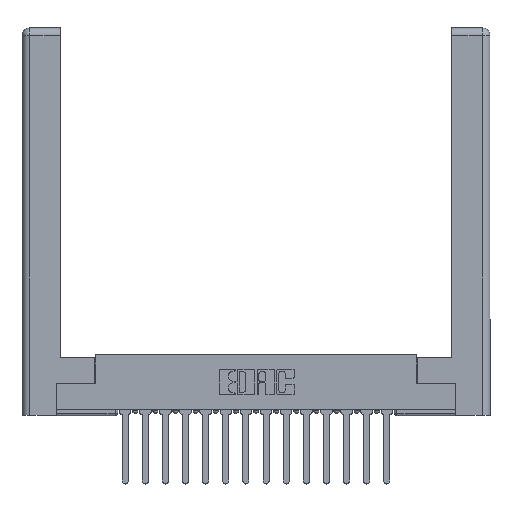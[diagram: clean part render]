
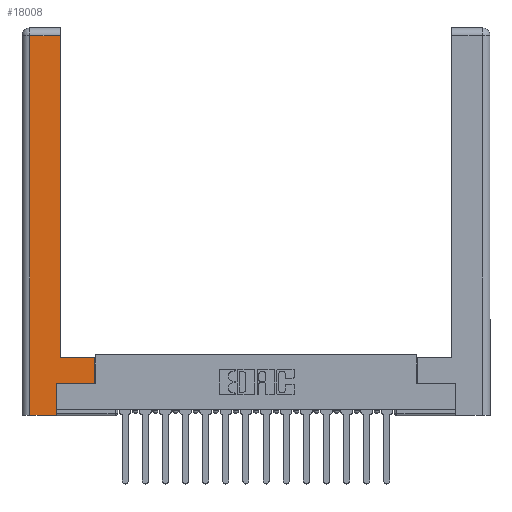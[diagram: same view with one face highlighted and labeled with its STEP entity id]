
A CAD part, top view. The second image highlights one B-rep face of the part: STEP entity #18008.
In plain terms, the highlighted planar face has unit normal (0, 0, 1).
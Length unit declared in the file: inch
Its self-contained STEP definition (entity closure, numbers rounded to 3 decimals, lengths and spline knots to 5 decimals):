
#327 = VERTEX_POINT ( 'NONE', #11752 ) ;
#416 = CARTESIAN_POINT ( 'NONE',  ( 0.0615, 0., 0. ) ) ;
#499 = ORIENTED_EDGE ( 'NONE', *, *, #4989, .T. ) ;
#632 = EDGE_CURVE ( 'NONE', #16639, #10606, #10550, .T. ) ;
#902 = ORIENTED_EDGE ( 'NONE', *, *, #17522, .T. ) ;
#1131 = CARTESIAN_POINT ( 'NONE',  ( 0.0615, 2.94, 0. ) ) ;
#1202 = DIRECTION ( 'NONE',  ( -1., 0., 0. ) ) ;
#1451 = ORIENTED_EDGE ( 'NONE', *, *, #632, .T. ) ;
#1500 = CARTESIAN_POINT ( 'NONE',  ( 0.565, 0.245, 0. ) ) ;
#1753 = DIRECTION ( 'NONE',  ( 1., 0., 0. ) ) ;
#1818 = CARTESIAN_POINT ( 'NONE',  ( 0.265, 0., 0. ) ) ;
#2394 = VECTOR ( 'NONE', #1753, 39.37008 ) ;
#2657 = PLANE ( 'NONE',  #8925 ) ;
#3227 = LINE ( 'NONE', #10267, #16869 ) ;
#3331 = CARTESIAN_POINT ( 'NONE',  ( 0.565, 0.245, 0. ) ) ;
#3826 = VERTEX_POINT ( 'NONE', #12232 ) ;
#3940 = LINE ( 'NONE', #14180, #14682 ) ;
#4027 = CARTESIAN_POINT ( 'NONE',  ( 0., 0., 0. ) ) ;
#4218 = VECTOR ( 'NONE', #5514, 39.37008 ) ;
#4342 = VECTOR ( 'NONE', #1202, 39.37008 ) ;
#4613 = DIRECTION ( 'NONE',  ( 0., 1., 0. ) ) ;
#4989 = EDGE_CURVE ( 'NONE', #12489, #15930, #3940, .T. ) ;
#5514 = DIRECTION ( 'NONE',  ( 1., 0., 0. ) ) ;
#5625 = EDGE_CURVE ( 'NONE', #16784, #3826, #3227, .T. ) ;
#5916 = EDGE_CURVE ( 'NONE', #327, #12489, #8117, .T. ) ;
#6084 = VECTOR ( 'NONE', #8935, 39.37008 ) ;
#6406 = DIRECTION ( 'NONE',  ( 0., 1., 0. ) ) ;
#8117 = LINE ( 'NONE', #15417, #4342 ) ;
#8521 = CARTESIAN_POINT ( 'NONE',  ( 0.295, 2.94, 0. ) ) ;
#8528 = FACE_OUTER_BOUND ( 'NONE', #9439, .T. ) ;
#8925 = AXIS2_PLACEMENT_3D ( 'NONE', #4027, #12835, #14040 ) ;
#8935 = DIRECTION ( 'NONE',  ( 0., -1., 0. ) ) ;
#8962 = VECTOR ( 'NONE', #4613, 39.37008 ) ;
#9422 = LINE ( 'NONE', #11675, #8962 ) ;
#9439 = EDGE_LOOP ( 'NONE', ( #499, #17723, #1451, #13150, #12830, #13193, #902, #9469 ) ) ;
#9469 = ORIENTED_EDGE ( 'NONE', *, *, #5916, .T. ) ;
#9688 = CARTESIAN_POINT ( 'NONE',  ( 0.0615, 0., 0. ) ) ;
#9830 = EDGE_CURVE ( 'NONE', #10606, #16784, #16957, .T. ) ;
#9956 = DIRECTION ( 'NONE',  ( 0., 1., 0. ) ) ;
#10267 = CARTESIAN_POINT ( 'NONE',  ( 0.265, 0.245, 0. ) ) ;
#10550 = LINE ( 'NONE', #9688, #6084 ) ;
#10606 = VERTEX_POINT ( 'NONE', #416 ) ;
#11515 = CARTESIAN_POINT ( 'NONE',  ( 0.0615, 2.94, 0. ) ) ;
#11533 = LINE ( 'NONE', #3331, #2394 ) ;
#11675 = CARTESIAN_POINT ( 'NONE',  ( 0.565, 0.45, 0. ) ) ;
#11752 = CARTESIAN_POINT ( 'NONE',  ( 0.565, 0.45, 0. ) ) ;
#11900 = LINE ( 'NONE', #1131, #13464 ) ;
#12232 = CARTESIAN_POINT ( 'NONE',  ( 0.265, 0.245, 0. ) ) ;
#12489 = VERTEX_POINT ( 'NONE', #15196 ) ;
#12830 = ORIENTED_EDGE ( 'NONE', *, *, #5625, .T. ) ;
#12835 = DIRECTION ( 'NONE',  ( 0., 0., -1. ) ) ;
#13150 = ORIENTED_EDGE ( 'NONE', *, *, #9830, .T. ) ;
#13193 = ORIENTED_EDGE ( 'NONE', *, *, #14957, .T. ) ;
#13464 = VECTOR ( 'NONE', #16766, 39.37008 ) ;
#14040 = DIRECTION ( 'NONE',  ( -1., 0., 0. ) ) ;
#14180 = CARTESIAN_POINT ( 'NONE',  ( 0.295, 3., 0. ) ) ;
#14682 = VECTOR ( 'NONE', #9956, 39.37008 ) ;
#14957 = EDGE_CURVE ( 'NONE', #3826, #16652, #11533, .T. ) ;
#15196 = CARTESIAN_POINT ( 'NONE',  ( 0.295, 0.45, 0. ) ) ;
#15417 = CARTESIAN_POINT ( 'NONE',  ( 0.295, 0.45, 0. ) ) ;
#15930 = VERTEX_POINT ( 'NONE', #8521 ) ;
#16639 = VERTEX_POINT ( 'NONE', #11515 ) ;
#16652 = VERTEX_POINT ( 'NONE', #1500 ) ;
#16766 = DIRECTION ( 'NONE',  ( -1., 0., 0. ) ) ;
#16784 = VERTEX_POINT ( 'NONE', #1818 ) ;
#16869 = VECTOR ( 'NONE', #6406, 39.37008 ) ;
#16957 = LINE ( 'NONE', #18511, #4218 ) ;
#17522 = EDGE_CURVE ( 'NONE', #16652, #327, #9422, .T. ) ;
#17723 = ORIENTED_EDGE ( 'NONE', *, *, #17995, .T. ) ;
#17995 = EDGE_CURVE ( 'NONE', #15930, #16639, #11900, .T. ) ;
#18008 = ADVANCED_FACE ( 'NONE', ( #8528 ), #2657, .F. ) ;
#18511 = CARTESIAN_POINT ( 'NONE',  ( 0.265, 0., 0. ) ) ;
